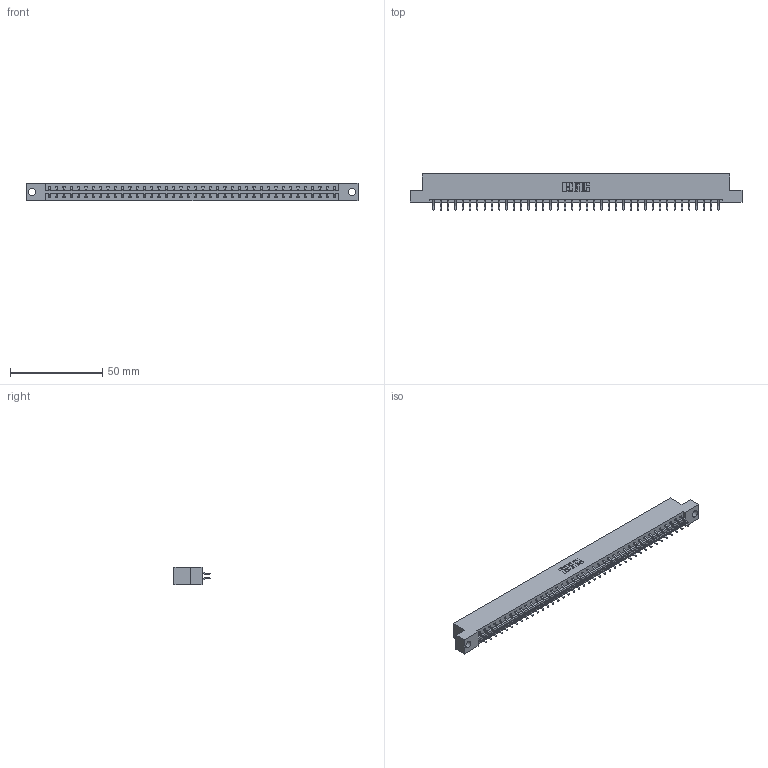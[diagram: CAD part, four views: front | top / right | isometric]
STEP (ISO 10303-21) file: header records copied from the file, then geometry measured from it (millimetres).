
FILE_DESCRIPTION (( 'STEP AP203' ), '1' );
FILE_NAME ('333-080-556-204.STEP', '2018-08-05T02:03:35', ( '' ), ( '' ), 'SwSTEP 2.0', 'SolidWorks 2016', '' );
FILE_SCHEMA (( 'CONFIG_CONTROL_DESIGN' ));
Length unit declared in the file: inch
Products named in the file (3): 333 Part_Flush - .156 Dia - TH; 345-292-001_556 Tail; 333-080-556-204
Assembly tree (81 placements, depth 2):
  333-080-556-204
    333 Part_Flush - .156 Dia - TH
    345-292-001_556 Tail  x80
Bounding box: 180.04 x 19.57 x 9.4 mm (x, y, z)
Volume: 18270.8 mm3; surface area: 21299.7 mm2
Topology: 81 solids, 81 shells, 4754 faces, 14151 edges, 9326 vertices
Faces by surface type: plane 3270, cylinder 1484
Entity records: 26215 total; most frequent: CARTESIAN_POINT 4362, ORIENTED_EDGE 4286, DIRECTION 3719, EDGE_CURVE 2143, LINE 2007, VECTOR 2007, VERTEX_POINT 1426, AXIS2_PLACEMENT_3D 856
